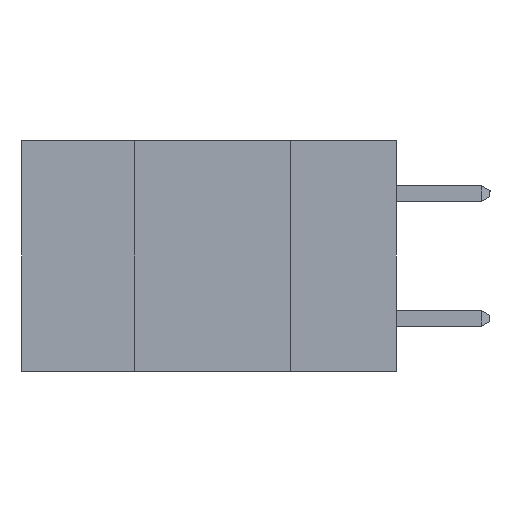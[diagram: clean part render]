
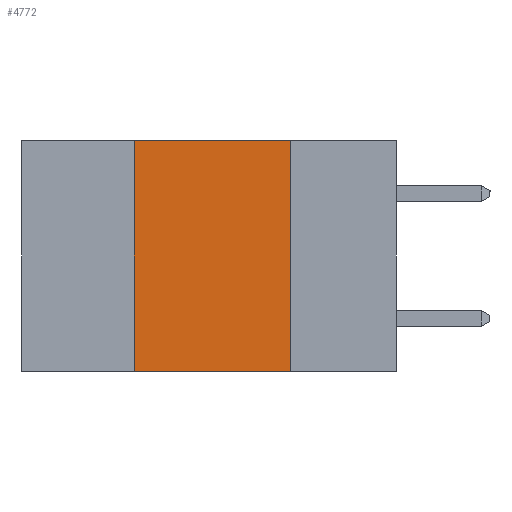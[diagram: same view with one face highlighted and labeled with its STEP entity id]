
A CAD part, left-side view. The second image highlights one B-rep face of the part: STEP entity #4772.
In plain terms, the highlighted planar face has unit normal (-1, 0, 0).
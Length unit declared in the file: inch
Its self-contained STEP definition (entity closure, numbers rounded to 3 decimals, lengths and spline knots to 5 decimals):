
#335 = CARTESIAN_POINT ( 'NONE',  ( 0., 0.6, 0. ) ) ;
#1465 = FACE_OUTER_BOUND ( 'NONE', #11151, .T. ) ;
#1714 = DIRECTION ( 'NONE',  ( 0., 0., -1. ) ) ;
#2478 = VECTOR ( 'NONE', #6808, 39.37008 ) ;
#2632 = DIRECTION ( 'NONE',  ( 1., 0., 0. ) ) ;
#3594 = EDGE_CURVE ( 'NONE', #4809, #10875, #15432, .T. ) ;
#4070 = ORIENTED_EDGE ( 'NONE', *, *, #3594, .F. ) ;
#4772 = ADVANCED_FACE ( 'NONE', ( #1465 ), #15545, .F. ) ;
#4809 = VERTEX_POINT ( 'NONE', #10525 ) ;
#4961 = LINE ( 'NONE', #7223, #12422 ) ;
#4963 = CARTESIAN_POINT ( 'NONE',  ( 0., 0.17, -0.37 ) ) ;
#4985 = VECTOR ( 'NONE', #12539, 39.37008 ) ;
#6808 = DIRECTION ( 'NONE',  ( 0., -1., 0. ) ) ;
#7223 = CARTESIAN_POINT ( 'NONE',  ( 0., 0.42, -0.37 ) ) ;
#7466 = AXIS2_PLACEMENT_3D ( 'NONE', #8085, #2632, #1714 ) ;
#8011 = LINE ( 'NONE', #13125, #4985 ) ;
#8085 = CARTESIAN_POINT ( 'NONE',  ( 0., 0.6, 0. ) ) ;
#8214 = ORIENTED_EDGE ( 'NONE', *, *, #14218, .T. ) ;
#8314 = CARTESIAN_POINT ( 'NONE',  ( 0., 0.17, 0. ) ) ;
#8828 = CARTESIAN_POINT ( 'NONE',  ( 0., 0.6, -0.37 ) ) ;
#10525 = CARTESIAN_POINT ( 'NONE',  ( 0., 0.42, 0. ) ) ;
#10875 = VERTEX_POINT ( 'NONE', #8314 ) ;
#10958 = EDGE_CURVE ( 'NONE', #11826, #4809, #4961, .T. ) ;
#11151 = EDGE_LOOP ( 'NONE', ( #14050, #4070, #15308, #8214 ) ) ;
#11826 = VERTEX_POINT ( 'NONE', #15021 ) ;
#12422 = VECTOR ( 'NONE', #13675, 39.37008 ) ;
#12539 = DIRECTION ( 'NONE',  ( 0., 0., -1. ) ) ;
#12693 = LINE ( 'NONE', #8828, #16197 ) ;
#13125 = CARTESIAN_POINT ( 'NONE',  ( 0., 0.17, -0.37 ) ) ;
#13675 = DIRECTION ( 'NONE',  ( 0., 0., 1. ) ) ;
#14050 = ORIENTED_EDGE ( 'NONE', *, *, #15302, .F. ) ;
#14218 = EDGE_CURVE ( 'NONE', #11826, #16039, #12693, .T. ) ;
#15021 = CARTESIAN_POINT ( 'NONE',  ( 0., 0.42, -0.37 ) ) ;
#15302 = EDGE_CURVE ( 'NONE', #10875, #16039, #8011, .T. ) ;
#15308 = ORIENTED_EDGE ( 'NONE', *, *, #10958, .F. ) ;
#15432 = LINE ( 'NONE', #335, #2478 ) ;
#15545 = PLANE ( 'NONE',  #7466 ) ;
#16039 = VERTEX_POINT ( 'NONE', #4963 ) ;
#16197 = VECTOR ( 'NONE', #16450, 39.37008 ) ;
#16450 = DIRECTION ( 'NONE',  ( 0., -1., 0. ) ) ;
